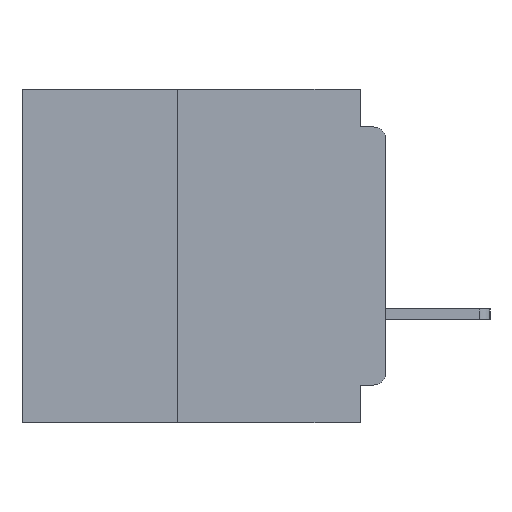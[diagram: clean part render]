
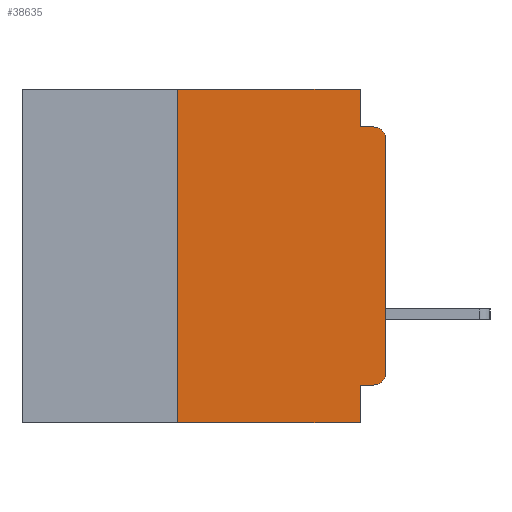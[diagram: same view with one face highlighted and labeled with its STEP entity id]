
A CAD part, left-side view. The second image highlights one B-rep face of the part: STEP entity #38635.
In plain terms, the highlighted planar face has unit normal (-1, 0, 0).
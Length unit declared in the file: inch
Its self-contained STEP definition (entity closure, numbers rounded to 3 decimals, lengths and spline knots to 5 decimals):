
#31 = CIRCLE ( 'NONE', #43183, 0.015 ) ;
#103 = DIRECTION ( 'NONE',  ( -1., 0., 0. ) ) ;
#966 = VECTOR ( 'NONE', #16875, 39.37008 ) ;
#1318 = DIRECTION ( 'NONE',  ( 0., 1., 0. ) ) ;
#1553 = ORIENTED_EDGE ( 'NONE', *, *, #35333, .T. ) ;
#2049 = DIRECTION ( 'NONE',  ( 0., 0., -1. ) ) ;
#2108 = EDGE_LOOP ( 'NONE', ( #26379, #1553, #49801, #27285, #3202, #30346, #22938, #24599, #29341, #24984 ) ) ;
#3202 = ORIENTED_EDGE ( 'NONE', *, *, #13413, .F. ) ;
#4129 = DIRECTION ( 'NONE',  ( -1., 0., 0. ) ) ;
#4396 = CIRCLE ( 'NONE', #47666, 0.015 ) ;
#5714 = CARTESIAN_POINT ( 'NONE',  ( 0., 0.437, 0. ) ) ;
#7831 = EDGE_CURVE ( 'NONE', #10076, #20079, #31, .T. ) ;
#8637 = VERTEX_POINT ( 'NONE', #30901 ) ;
#9895 = CARTESIAN_POINT ( 'NONE',  ( 0., 0.031, -0.4 ) ) ;
#9908 = DIRECTION ( 'NONE',  ( 0., 0., -1. ) ) ;
#10076 = VERTEX_POINT ( 'NONE', #17069 ) ;
#12352 = VECTOR ( 'NONE', #22737, 39.37008 ) ;
#13032 = CARTESIAN_POINT ( 'NONE',  ( 0., 0.25, -0.4 ) ) ;
#13413 = EDGE_CURVE ( 'NONE', #39185, #29514, #38035, .T. ) ;
#14030 = CARTESIAN_POINT ( 'NONE',  ( 0., 0.25, 0. ) ) ;
#14564 = DIRECTION ( 'NONE',  ( 0., 0., -1. ) ) ;
#15295 = VERTEX_POINT ( 'NONE', #9895 ) ;
#16875 = DIRECTION ( 'NONE',  ( 0., -1., 0. ) ) ;
#17069 = CARTESIAN_POINT ( 'NONE',  ( 0., 0.015, -0.355 ) ) ;
#17236 = DIRECTION ( 'NONE',  ( 0., -1., 0. ) ) ;
#19485 = VECTOR ( 'NONE', #14564, 39.37008 ) ;
#20079 = VERTEX_POINT ( 'NONE', #49717 ) ;
#20210 = FACE_OUTER_BOUND ( 'NONE', #2108, .T. ) ;
#20369 = LINE ( 'NONE', #40265, #30119 ) ;
#21145 = EDGE_CURVE ( 'NONE', #10076, #34851, #36281, .T. ) ;
#22737 = DIRECTION ( 'NONE',  ( 0., 0., 1. ) ) ;
#22797 = CARTESIAN_POINT ( 'NONE',  ( 0., 0.031, -0.355 ) ) ;
#22938 = ORIENTED_EDGE ( 'NONE', *, *, #36459, .T. ) ;
#23357 = LINE ( 'NONE', #47497, #12352 ) ;
#23954 = AXIS2_PLACEMENT_3D ( 'NONE', #5714, #34720, #9908 ) ;
#24599 = ORIENTED_EDGE ( 'NONE', *, *, #42601, .F. ) ;
#24954 = CARTESIAN_POINT ( 'NONE',  ( 0., 0.015, -0.34 ) ) ;
#24984 = ORIENTED_EDGE ( 'NONE', *, *, #7831, .T. ) ;
#25236 = VECTOR ( 'NONE', #1318, 39.37008 ) ;
#26379 = ORIENTED_EDGE ( 'NONE', *, *, #27220, .T. ) ;
#26397 = PLANE ( 'NONE',  #23954 ) ;
#26814 = CARTESIAN_POINT ( 'NONE',  ( 0., 0.031, -0.045 ) ) ;
#27220 = EDGE_CURVE ( 'NONE', #20079, #52170, #33047, .T. ) ;
#27285 = ORIENTED_EDGE ( 'NONE', *, *, #39268, .F. ) ;
#28735 = CARTESIAN_POINT ( 'NONE',  ( 0., 0.031, 0. ) ) ;
#28993 = CARTESIAN_POINT ( 'NONE',  ( 0., 0.015, -0.06 ) ) ;
#29158 = DIRECTION ( 'NONE',  ( 0., 0., -1. ) ) ;
#29341 = ORIENTED_EDGE ( 'NONE', *, *, #21145, .F. ) ;
#29514 = VERTEX_POINT ( 'NONE', #28735 ) ;
#30119 = VECTOR ( 'NONE', #52706, 39.37008 ) ;
#30314 = LINE ( 'NONE', #51628, #38668 ) ;
#30346 = ORIENTED_EDGE ( 'NONE', *, *, #40784, .F. ) ;
#30521 = LINE ( 'NONE', #51960, #19485 ) ;
#30901 = CARTESIAN_POINT ( 'NONE',  ( 0., 0.015, -0.045 ) ) ;
#33047 = LINE ( 'NONE', #33158, #53679 ) ;
#33111 = DIRECTION ( 'NONE',  ( 0., 0., -1. ) ) ;
#33158 = CARTESIAN_POINT ( 'NONE',  ( 0., 0., 0. ) ) ;
#34326 = CARTESIAN_POINT ( 'NONE',  ( 0., 0., -0.355 ) ) ;
#34720 = DIRECTION ( 'NONE',  ( 1., 0., 0. ) ) ;
#34851 = VERTEX_POINT ( 'NONE', #22797 ) ;
#35333 = EDGE_CURVE ( 'NONE', #52170, #8637, #4396, .T. ) ;
#36281 = LINE ( 'NONE', #34326, #25236 ) ;
#36459 = EDGE_CURVE ( 'NONE', #41796, #15295, #43775, .T. ) ;
#37312 = DIRECTION ( 'NONE',  ( 0., 0., 1. ) ) ;
#37862 = CARTESIAN_POINT ( 'NONE',  ( 0., 0.437, 0. ) ) ;
#38035 = LINE ( 'NONE', #37862, #47733 ) ;
#38635 = ADVANCED_FACE ( 'NONE', ( #20210 ), #26397, .F. ) ;
#38668 = VECTOR ( 'NONE', #2049, 39.37008 ) ;
#39185 = VERTEX_POINT ( 'NONE', #14030 ) ;
#39268 = EDGE_CURVE ( 'NONE', #29514, #46632, #30521, .T. ) ;
#40265 = CARTESIAN_POINT ( 'NONE',  ( 0., 0., -0.045 ) ) ;
#40784 = EDGE_CURVE ( 'NONE', #41796, #39185, #23357, .T. ) ;
#41653 = CARTESIAN_POINT ( 'NONE',  ( 0., 0.437, -0.4 ) ) ;
#41796 = VERTEX_POINT ( 'NONE', #13032 ) ;
#42601 = EDGE_CURVE ( 'NONE', #34851, #15295, #30314, .T. ) ;
#43183 = AXIS2_PLACEMENT_3D ( 'NONE', #24954, #103, #29158 ) ;
#43775 = LINE ( 'NONE', #41653, #966 ) ;
#46632 = VERTEX_POINT ( 'NONE', #26814 ) ;
#47426 = EDGE_CURVE ( 'NONE', #46632, #8637, #20369, .T. ) ;
#47497 = CARTESIAN_POINT ( 'NONE',  ( 0., 0.25, -0.4 ) ) ;
#47666 = AXIS2_PLACEMENT_3D ( 'NONE', #28993, #4129, #33111 ) ;
#47733 = VECTOR ( 'NONE', #17236, 39.37008 ) ;
#49387 = CARTESIAN_POINT ( 'NONE',  ( 0., 0., -0.06 ) ) ;
#49717 = CARTESIAN_POINT ( 'NONE',  ( 0., 0., -0.34 ) ) ;
#49801 = ORIENTED_EDGE ( 'NONE', *, *, #47426, .F. ) ;
#51628 = CARTESIAN_POINT ( 'NONE',  ( 0., 0.031, -0.4 ) ) ;
#51960 = CARTESIAN_POINT ( 'NONE',  ( 0., 0.031, 0. ) ) ;
#52170 = VERTEX_POINT ( 'NONE', #49387 ) ;
#52706 = DIRECTION ( 'NONE',  ( 0., -1., 0. ) ) ;
#53679 = VECTOR ( 'NONE', #37312, 39.37008 ) ;
